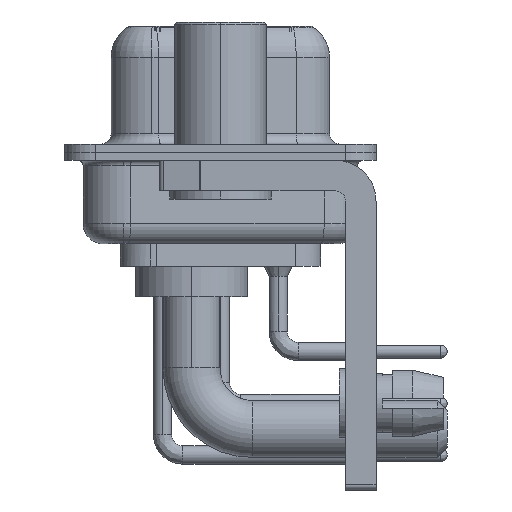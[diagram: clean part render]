
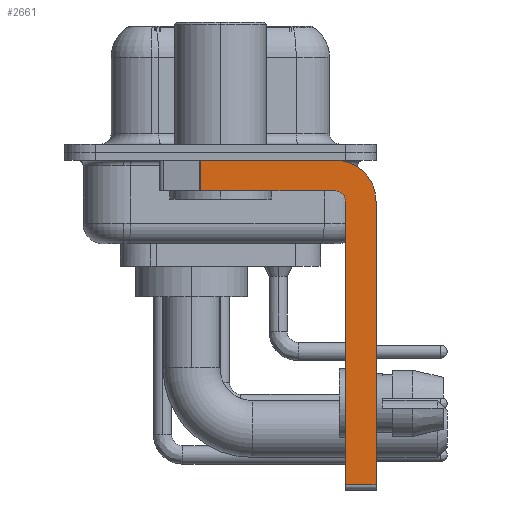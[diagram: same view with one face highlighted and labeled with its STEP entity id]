
A CAD part, left-side view. The second image highlights one B-rep face of the part: STEP entity #2661.
In plain terms, the highlighted planar face has unit normal (-1, 0, 0).
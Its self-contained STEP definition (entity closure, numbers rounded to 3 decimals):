
#328 = DIRECTION ( 'NONE',  ( 0., 0., 1. ) ) ;
#1077 = DIRECTION ( 'NONE',  ( 0., 0., -1. ) ) ;
#2661 = ADVANCED_FACE ( 'NONE', ( #25918 ), #14523, .F. ) ;
#3653 = CARTESIAN_POINT ( 'NONE',  ( -2.9, 0.978, -1.9 ) ) ;
#3929 = LINE ( 'NONE', #18353, #4740 ) ;
#4740 = VECTOR ( 'NONE', #15506, 1000. ) ;
#7012 = DIRECTION ( 'NONE',  ( 0., -1., 0. ) ) ;
#7052 = VECTOR ( 'NONE', #35822, 1000. ) ;
#7256 = ORIENTED_EDGE ( 'NONE', *, *, #14449, .F. ) ;
#9003 = DIRECTION ( 'NONE',  ( 0., 0., -1. ) ) ;
#9486 = LINE ( 'NONE', #12355, #35711 ) ;
#9985 = EDGE_CURVE ( 'NONE', #23545, #20023, #10282, .T. ) ;
#10282 = LINE ( 'NONE', #21684, #20765 ) ;
#10580 = EDGE_CURVE ( 'NONE', #32188, #28556, #14716, .T. ) ;
#11738 = CARTESIAN_POINT ( 'NONE',  ( -2.9, -5.65, -2.4 ) ) ;
#12033 = LINE ( 'NONE', #32695, #30170 ) ;
#12294 = CIRCLE ( 'NONE', #35281, 0.5 ) ;
#12355 = CARTESIAN_POINT ( 'NONE',  ( -2.9, 3., -0.4 ) ) ;
#12697 = CARTESIAN_POINT ( 'NONE',  ( -2.9, -7.65, -2.4 ) ) ;
#14449 = EDGE_CURVE ( 'NONE', #37236, #28556, #30533, .T. ) ;
#14523 = PLANE ( 'NONE',  #25991 ) ;
#14716 = LINE ( 'NONE', #29139, #34094 ) ;
#15506 = DIRECTION ( 'NONE',  ( 0., 0., 1. ) ) ;
#16165 = CARTESIAN_POINT ( 'NONE',  ( -2.9, -5.65, -1.9 ) ) ;
#17013 = CARTESIAN_POINT ( 'NONE',  ( -2.9, -7.65, -16.35 ) ) ;
#18079 = CARTESIAN_POINT ( 'NONE',  ( -2.9, -5.65, -0.4 ) ) ;
#18353 = CARTESIAN_POINT ( 'NONE',  ( -2.9, -6.15, -16.6 ) ) ;
#18918 = EDGE_CURVE ( 'NONE', #32188, #22115, #9486, .T. ) ;
#20023 = VERTEX_POINT ( 'NONE', #17013 ) ;
#20176 = CIRCLE ( 'NONE', #20773, 2. ) ;
#20765 = VECTOR ( 'NONE', #25089, 1000. ) ;
#20773 = AXIS2_PLACEMENT_3D ( 'NONE', #36179, #30887, #1077 ) ;
#21107 = VERTEX_POINT ( 'NONE', #37007 ) ;
#21684 = CARTESIAN_POINT ( 'NONE',  ( -2.9, -7.65, -2.4 ) ) ;
#22115 = VERTEX_POINT ( 'NONE', #18079 ) ;
#22425 = ORIENTED_EDGE ( 'NONE', *, *, #10580, .T. ) ;
#22815 = CARTESIAN_POINT ( 'NONE',  ( -2.9, 0.978, -0.4 ) ) ;
#23545 = VERTEX_POINT ( 'NONE', #12697 ) ;
#23878 = DIRECTION ( 'NONE',  ( -1., 0., 0. ) ) ;
#24162 = ORIENTED_EDGE ( 'NONE', *, *, #9985, .F. ) ;
#24557 = EDGE_LOOP ( 'NONE', ( #30759, #22425, #7256, #26194, #28891, #36277, #24162, #29711 ) ) ;
#25089 = DIRECTION ( 'NONE',  ( 0., 0., -1. ) ) ;
#25612 = EDGE_CURVE ( 'NONE', #36340, #20023, #12033, .T. ) ;
#25739 = DIRECTION ( 'NONE',  ( 1., 0., 0. ) ) ;
#25918 = FACE_OUTER_BOUND ( 'NONE', #24557, .T. ) ;
#25991 = AXIS2_PLACEMENT_3D ( 'NONE', #31780, #25739, #9003 ) ;
#26194 = ORIENTED_EDGE ( 'NONE', *, *, #30999, .F. ) ;
#27087 = EDGE_CURVE ( 'NONE', #36340, #21107, #3929, .T. ) ;
#28556 = VERTEX_POINT ( 'NONE', #3653 ) ;
#28891 = ORIENTED_EDGE ( 'NONE', *, *, #27087, .F. ) ;
#29139 = CARTESIAN_POINT ( 'NONE',  ( -2.9, 0.978, -1.9 ) ) ;
#29711 = ORIENTED_EDGE ( 'NONE', *, *, #31203, .F. ) ;
#30170 = VECTOR ( 'NONE', #35346, 1000. ) ;
#30533 = LINE ( 'NONE', #35635, #7052 ) ;
#30759 = ORIENTED_EDGE ( 'NONE', *, *, #18918, .F. ) ;
#30887 = DIRECTION ( 'NONE',  ( 1., 0., 0. ) ) ;
#30999 = EDGE_CURVE ( 'NONE', #21107, #37236, #12294, .T. ) ;
#31203 = EDGE_CURVE ( 'NONE', #22115, #23545, #20176, .T. ) ;
#31780 = CARTESIAN_POINT ( 'NONE',  ( -2.9, -5.65, -2.4 ) ) ;
#32188 = VERTEX_POINT ( 'NONE', #22815 ) ;
#32695 = CARTESIAN_POINT ( 'NONE',  ( -2.9, -5.65, -16.35 ) ) ;
#34037 = CARTESIAN_POINT ( 'NONE',  ( -2.9, -6.15, -16.35 ) ) ;
#34094 = VECTOR ( 'NONE', #34806, 1000. ) ;
#34806 = DIRECTION ( 'NONE',  ( 0., 0., -1. ) ) ;
#35281 = AXIS2_PLACEMENT_3D ( 'NONE', #11738, #23878, #328 ) ;
#35346 = DIRECTION ( 'NONE',  ( 0., -1., 0. ) ) ;
#35635 = CARTESIAN_POINT ( 'NONE',  ( -2.9, -5.65, -1.9 ) ) ;
#35711 = VECTOR ( 'NONE', #7012, 1000. ) ;
#35822 = DIRECTION ( 'NONE',  ( 0., 1., 0. ) ) ;
#36179 = CARTESIAN_POINT ( 'NONE',  ( -2.9, -5.65, -2.4 ) ) ;
#36277 = ORIENTED_EDGE ( 'NONE', *, *, #25612, .T. ) ;
#36340 = VERTEX_POINT ( 'NONE', #34037 ) ;
#37007 = CARTESIAN_POINT ( 'NONE',  ( -2.9, -6.15, -2.4 ) ) ;
#37236 = VERTEX_POINT ( 'NONE', #16165 ) ;
